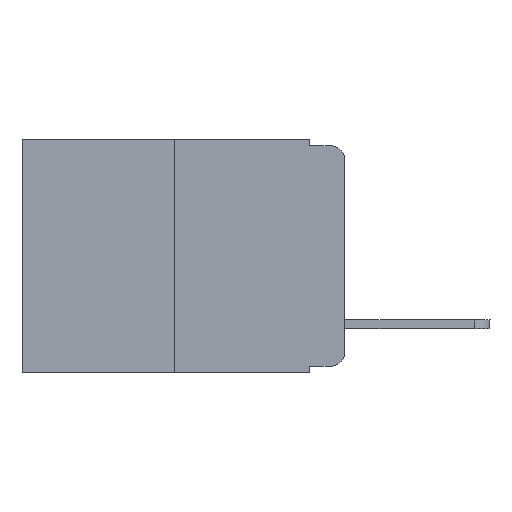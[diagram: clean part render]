
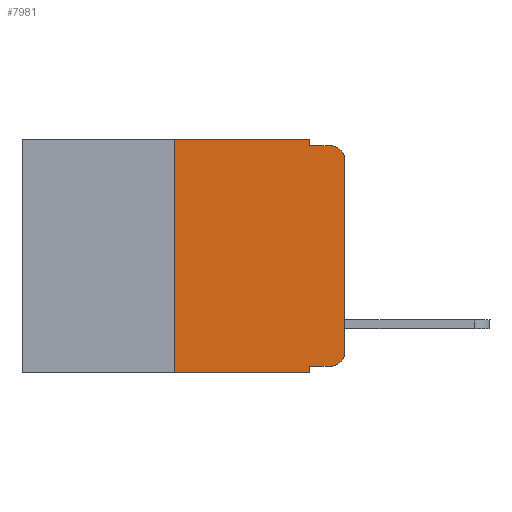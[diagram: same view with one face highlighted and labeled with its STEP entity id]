
A CAD part, left-side view. The second image highlights one B-rep face of the part: STEP entity #7981.
In plain terms, the highlighted planar face has unit normal (-1, 0, 0).
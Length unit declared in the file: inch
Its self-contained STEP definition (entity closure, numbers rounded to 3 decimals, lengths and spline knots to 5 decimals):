
#180 = AXIS2_PLACEMENT_3D ( 'NONE', #877, #9102, #2593 ) ;
#250 = VECTOR ( 'NONE', #7951, 39.37008 ) ;
#524 = CARTESIAN_POINT ( 'NONE',  ( 0., 0.051, -0.01 ) ) ;
#572 = EDGE_CURVE ( 'NONE', #3290, #6091, #1399, .T. ) ;
#621 = LINE ( 'NONE', #9083, #8280 ) ;
#877 = CARTESIAN_POINT ( 'NONE',  ( 0., 0.02, -0.313 ) ) ;
#933 = EDGE_CURVE ( 'NONE', #8012, #6091, #1451, .T. ) ;
#1047 = ORIENTED_EDGE ( 'NONE', *, *, #933, .F. ) ;
#1258 = CARTESIAN_POINT ( 'NONE',  ( 0., 0.02, -0.01 ) ) ;
#1399 = CIRCLE ( 'NONE', #1574, 0.02 ) ;
#1451 = LINE ( 'NONE', #524, #9641 ) ;
#1541 = CARTESIAN_POINT ( 'NONE',  ( 0., 0.051, 0. ) ) ;
#1574 = AXIS2_PLACEMENT_3D ( 'NONE', #10760, #2276, #8904 ) ;
#1592 = EDGE_CURVE ( 'NONE', #9765, #4464, #12152, .T. ) ;
#1669 = EDGE_CURVE ( 'NONE', #9943, #7122, #3434, .T. ) ;
#1693 = DIRECTION ( 'NONE',  ( 0., 0., 1. ) ) ;
#2028 = DIRECTION ( 'NONE',  ( 0., 0., -1. ) ) ;
#2080 = ORIENTED_EDGE ( 'NONE', *, *, #6602, .T. ) ;
#2139 = VERTEX_POINT ( 'NONE', #9340 ) ;
#2276 = DIRECTION ( 'NONE',  ( -1., 0., 0. ) ) ;
#2398 = ORIENTED_EDGE ( 'NONE', *, *, #5005, .F. ) ;
#2539 = VECTOR ( 'NONE', #10263, 39.37008 ) ;
#2575 = DIRECTION ( 'NONE',  ( 0., 0., -1. ) ) ;
#2593 = DIRECTION ( 'NONE',  ( 0., 0., -1. ) ) ;
#2820 = DIRECTION ( 'NONE',  ( 1., 0., 0. ) ) ;
#2877 = FACE_OUTER_BOUND ( 'NONE', #7485, .T. ) ;
#2905 = ORIENTED_EDGE ( 'NONE', *, *, #6168, .T. ) ;
#2945 = CARTESIAN_POINT ( 'NONE',  ( 0., 0.051, -0.01 ) ) ;
#3290 = VERTEX_POINT ( 'NONE', #10956 ) ;
#3434 = LINE ( 'NONE', #8891, #250 ) ;
#3820 = DIRECTION ( 'NONE',  ( 0., -1., 0. ) ) ;
#3954 = LINE ( 'NONE', #8826, #8640 ) ;
#4123 = VECTOR ( 'NONE', #1693, 39.37008 ) ;
#4374 = LINE ( 'NONE', #8368, #4123 ) ;
#4464 = VERTEX_POINT ( 'NONE', #6641 ) ;
#4481 = DIRECTION ( 'NONE',  ( 0., -1., 0. ) ) ;
#4561 = ORIENTED_EDGE ( 'NONE', *, *, #5654, .F. ) ;
#4663 = DIRECTION ( 'NONE',  ( 0., -1., 0. ) ) ;
#4670 = PLANE ( 'NONE',  #6678 ) ;
#4784 = VECTOR ( 'NONE', #4663, 39.37008 ) ;
#4794 = CARTESIAN_POINT ( 'NONE',  ( 0., 0.051, -0.333 ) ) ;
#4826 = ORIENTED_EDGE ( 'NONE', *, *, #8310, .T. ) ;
#4991 = ORIENTED_EDGE ( 'NONE', *, *, #1592, .T. ) ;
#5005 = EDGE_CURVE ( 'NONE', #7122, #11173, #3954, .T. ) ;
#5210 = ORIENTED_EDGE ( 'NONE', *, *, #572, .T. ) ;
#5419 = LINE ( 'NONE', #12153, #5685 ) ;
#5654 = EDGE_CURVE ( 'NONE', #9765, #2139, #5419, .T. ) ;
#5685 = VECTOR ( 'NONE', #2575, 39.37008 ) ;
#5701 = CIRCLE ( 'NONE', #180, 0.02 ) ;
#5900 = ORIENTED_EDGE ( 'NONE', *, *, #6232, .F. ) ;
#6091 = VERTEX_POINT ( 'NONE', #1258 ) ;
#6168 = EDGE_CURVE ( 'NONE', #4464, #8845, #5701, .T. ) ;
#6232 = EDGE_CURVE ( 'NONE', #11173, #8012, #12112, .T. ) ;
#6602 = EDGE_CURVE ( 'NONE', #9943, #2139, #621, .T. ) ;
#6641 = CARTESIAN_POINT ( 'NONE',  ( 0., 0.02, -0.333 ) ) ;
#6678 = AXIS2_PLACEMENT_3D ( 'NONE', #7557, #2820, #2028 ) ;
#7122 = VERTEX_POINT ( 'NONE', #8054 ) ;
#7435 = CARTESIAN_POINT ( 'NONE',  ( 0., 0.051, -0.333 ) ) ;
#7485 = EDGE_LOOP ( 'NONE', ( #4826, #5210, #1047, #5900, #2398, #9327, #2080, #4561, #4991, #2905 ) ) ;
#7532 = CARTESIAN_POINT ( 'NONE',  ( 0., 0., -0.313 ) ) ;
#7557 = CARTESIAN_POINT ( 'NONE',  ( 0., 0.473, 0. ) ) ;
#7951 = DIRECTION ( 'NONE',  ( 0., 0., 1. ) ) ;
#7981 = ADVANCED_FACE ( 'NONE', ( #2877 ), #4670, .F. ) ;
#8012 = VERTEX_POINT ( 'NONE', #2945 ) ;
#8054 = CARTESIAN_POINT ( 'NONE',  ( 0., 0.25, 0. ) ) ;
#8280 = VECTOR ( 'NONE', #4481, 39.37008 ) ;
#8310 = EDGE_CURVE ( 'NONE', #8845, #3290, #4374, .T. ) ;
#8368 = CARTESIAN_POINT ( 'NONE',  ( 0., 0., 0. ) ) ;
#8640 = VECTOR ( 'NONE', #3820, 39.37008 ) ;
#8723 = CARTESIAN_POINT ( 'NONE',  ( 0., 0.25, -0.343 ) ) ;
#8826 = CARTESIAN_POINT ( 'NONE',  ( 0., 0.473, 0. ) ) ;
#8845 = VERTEX_POINT ( 'NONE', #7532 ) ;
#8891 = CARTESIAN_POINT ( 'NONE',  ( 0., 0.25, 0. ) ) ;
#8904 = DIRECTION ( 'NONE',  ( 0., 0., -1. ) ) ;
#9036 = DIRECTION ( 'NONE',  ( 0., -1., 0. ) ) ;
#9083 = CARTESIAN_POINT ( 'NONE',  ( 0., 0.473, -0.343 ) ) ;
#9102 = DIRECTION ( 'NONE',  ( -1., 0., 0. ) ) ;
#9327 = ORIENTED_EDGE ( 'NONE', *, *, #1669, .F. ) ;
#9340 = CARTESIAN_POINT ( 'NONE',  ( 0., 0.051, -0.343 ) ) ;
#9641 = VECTOR ( 'NONE', #9036, 39.37008 ) ;
#9765 = VERTEX_POINT ( 'NONE', #4794 ) ;
#9943 = VERTEX_POINT ( 'NONE', #8723 ) ;
#10263 = DIRECTION ( 'NONE',  ( 0., 0., -1. ) ) ;
#10760 = CARTESIAN_POINT ( 'NONE',  ( 0., 0.02, -0.03 ) ) ;
#10956 = CARTESIAN_POINT ( 'NONE',  ( 0., 0., -0.03 ) ) ;
#11173 = VERTEX_POINT ( 'NONE', #11791 ) ;
#11791 = CARTESIAN_POINT ( 'NONE',  ( 0., 0.051, 0. ) ) ;
#12112 = LINE ( 'NONE', #1541, #2539 ) ;
#12152 = LINE ( 'NONE', #7435, #4784 ) ;
#12153 = CARTESIAN_POINT ( 'NONE',  ( 0., 0.051, 0. ) ) ;
